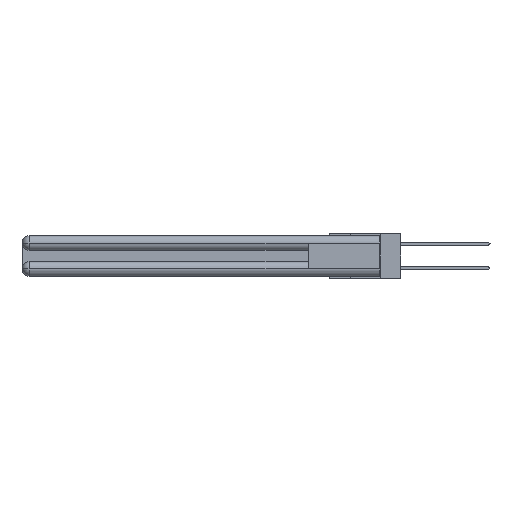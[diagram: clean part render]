
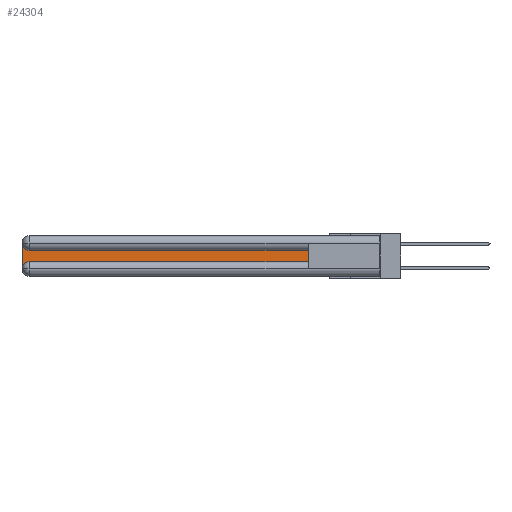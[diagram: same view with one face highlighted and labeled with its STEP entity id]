
A CAD part, left-side view. The second image highlights one B-rep face of the part: STEP entity #24304.
In plain terms, the highlighted planar face has unit normal (-1, 0, 0).
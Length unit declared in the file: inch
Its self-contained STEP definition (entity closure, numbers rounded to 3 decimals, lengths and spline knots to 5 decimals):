
#411 = EDGE_LOOP ( 'NONE', ( #8263, #2927, #6430, #22804, #9240, #7419 ) ) ;
#623 = VECTOR ( 'NONE', #10914, 39.37008 ) ;
#735 = LINE ( 'NONE', #5919, #25553 ) ;
#1487 = CIRCLE ( 'NONE', #31794, 0.06 ) ;
#1608 = DIRECTION ( 'NONE',  ( 0., 0., -1. ) ) ;
#2927 = ORIENTED_EDGE ( 'NONE', *, *, #29864, .T. ) ;
#3285 = VERTEX_POINT ( 'NONE', #7117 ) ;
#3434 = CARTESIAN_POINT ( 'NONE',  ( 0.075, 3., -0.1225 ) ) ;
#3518 = CARTESIAN_POINT ( 'NONE',  ( 0.075, 3., -0.2775 ) ) ;
#3577 = EDGE_CURVE ( 'NONE', #10641, #25248, #31234, .T. ) ;
#3775 = CARTESIAN_POINT ( 'NONE',  ( 0.075, 2.94, -0.2775 ) ) ;
#4932 = CIRCLE ( 'NONE', #16575, 0.06 ) ;
#5365 = DIRECTION ( 'NONE',  ( 0., 0., -1. ) ) ;
#5919 = CARTESIAN_POINT ( 'NONE',  ( 0.075, 0.6, -0.2175 ) ) ;
#6430 = ORIENTED_EDGE ( 'NONE', *, *, #3577, .T. ) ;
#7117 = CARTESIAN_POINT ( 'NONE',  ( 0.075, 2.94, -0.2175 ) ) ;
#7247 = CARTESIAN_POINT ( 'NONE',  ( 0.075, 0.6, -0.2175 ) ) ;
#7419 = ORIENTED_EDGE ( 'NONE', *, *, #15864, .T. ) ;
#7685 = DIRECTION ( 'NONE',  ( 0., 1., 0. ) ) ;
#8263 = ORIENTED_EDGE ( 'NONE', *, *, #17017, .T. ) ;
#8437 = CARTESIAN_POINT ( 'NONE',  ( 0.075, 0.6, -0.2175 ) ) ;
#9042 = VECTOR ( 'NONE', #11756, 39.37008 ) ;
#9240 = ORIENTED_EDGE ( 'NONE', *, *, #22465, .T. ) ;
#10641 = VERTEX_POINT ( 'NONE', #17626 ) ;
#10656 = LINE ( 'NONE', #8437, #623 ) ;
#10914 = DIRECTION ( 'NONE',  ( 0., 0., 1. ) ) ;
#11756 = DIRECTION ( 'NONE',  ( 0., 0., -1. ) ) ;
#12677 = CARTESIAN_POINT ( 'NONE',  ( 0.075, 0.6, -0.1225 ) ) ;
#14142 = EDGE_CURVE ( 'NONE', #25248, #3285, #4932, .T. ) ;
#15061 = CARTESIAN_POINT ( 'NONE',  ( 0.075, 0.6, -0.1225 ) ) ;
#15864 = EDGE_CURVE ( 'NONE', #31358, #17038, #10656, .T. ) ;
#15886 = VERTEX_POINT ( 'NONE', #20840 ) ;
#16575 = AXIS2_PLACEMENT_3D ( 'NONE', #3775, #28711, #1608 ) ;
#17017 = EDGE_CURVE ( 'NONE', #17038, #15886, #27980, .T. ) ;
#17038 = VERTEX_POINT ( 'NONE', #12677 ) ;
#17536 = CARTESIAN_POINT ( 'NONE',  ( 0.075, 2.94, -0.0625 ) ) ;
#17626 = CARTESIAN_POINT ( 'NONE',  ( 0.075, 3., -0.0625 ) ) ;
#19368 = CARTESIAN_POINT ( 'NONE',  ( 0.075, 3., -0.2175 ) ) ;
#20840 = CARTESIAN_POINT ( 'NONE',  ( 0.075, 2.94, -0.1225 ) ) ;
#22230 = FACE_OUTER_BOUND ( 'NONE', #411, .T. ) ;
#22465 = EDGE_CURVE ( 'NONE', #3285, #31358, #735, .T. ) ;
#22804 = ORIENTED_EDGE ( 'NONE', *, *, #14142, .T. ) ;
#24098 = VECTOR ( 'NONE', #7685, 39.37008 ) ;
#24304 = ADVANCED_FACE ( 'NONE', ( #22230 ), #30679, .F. ) ;
#25248 = VERTEX_POINT ( 'NONE', #3518 ) ;
#25467 = DIRECTION ( 'NONE',  ( 1., 0., 0. ) ) ;
#25539 = DIRECTION ( 'NONE',  ( 1., 0., 0. ) ) ;
#25553 = VECTOR ( 'NONE', #30361, 39.37008 ) ;
#27329 = DIRECTION ( 'NONE',  ( 0., 0., -1. ) ) ;
#27980 = LINE ( 'NONE', #15061, #24098 ) ;
#28711 = DIRECTION ( 'NONE',  ( 1., 0., 0. ) ) ;
#29864 = EDGE_CURVE ( 'NONE', #15886, #10641, #1487, .T. ) ;
#30026 = AXIS2_PLACEMENT_3D ( 'NONE', #3434, #25539, #5365 ) ;
#30361 = DIRECTION ( 'NONE',  ( 0., -1., 0. ) ) ;
#30679 = PLANE ( 'NONE',  #30026 ) ;
#31234 = LINE ( 'NONE', #19368, #9042 ) ;
#31358 = VERTEX_POINT ( 'NONE', #7247 ) ;
#31794 = AXIS2_PLACEMENT_3D ( 'NONE', #17536, #25467, #27329 ) ;
